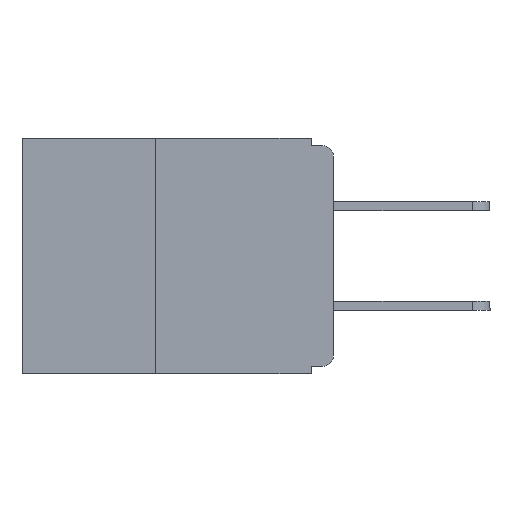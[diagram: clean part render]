
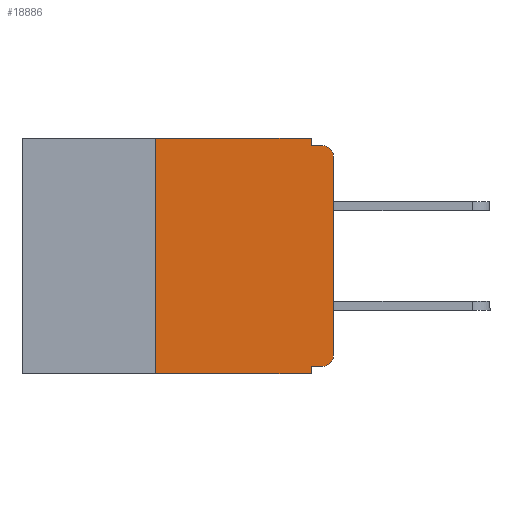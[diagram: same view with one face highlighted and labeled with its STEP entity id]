
A CAD part, left-side view. The second image highlights one B-rep face of the part: STEP entity #18886.
In plain terms, the highlighted planar face has unit normal (-1, 0, 0).
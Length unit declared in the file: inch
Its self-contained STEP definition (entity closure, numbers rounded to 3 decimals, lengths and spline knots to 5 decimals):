
#1476 = EDGE_CURVE ( 'NONE', #25379, #18260, #19982, .T. ) ;
#1733 = VECTOR ( 'NONE', #20077, 39.37008 ) ;
#2137 = CARTESIAN_POINT ( 'NONE',  ( 0., 0.015, -0.025 ) ) ;
#2163 = ORIENTED_EDGE ( 'NONE', *, *, #23606, .F. ) ;
#2522 = ORIENTED_EDGE ( 'NONE', *, *, #3370, .T. ) ;
#3039 = ORIENTED_EDGE ( 'NONE', *, *, #7966, .T. ) ;
#3225 = LINE ( 'NONE', #8152, #17034 ) ;
#3334 = ORIENTED_EDGE ( 'NONE', *, *, #30245, .F. ) ;
#3370 = EDGE_CURVE ( 'NONE', #20870, #31710, #18182, .T. ) ;
#4923 = DIRECTION ( 'NONE',  ( 0., 0., -1. ) ) ;
#5329 = DIRECTION ( 'NONE',  ( 0., 1., 0. ) ) ;
#5519 = DIRECTION ( 'NONE',  ( 0., -1., 0. ) ) ;
#5835 = CARTESIAN_POINT ( 'NONE',  ( 0., 0.437, 0. ) ) ;
#5844 = CARTESIAN_POINT ( 'NONE',  ( 0., 0.25, 0. ) ) ;
#5869 = ORIENTED_EDGE ( 'NONE', *, *, #1476, .F. ) ;
#5966 = VECTOR ( 'NONE', #34291, 39.37008 ) ;
#7051 = CARTESIAN_POINT ( 'NONE',  ( 0., 0.25, -0.33 ) ) ;
#7355 = DIRECTION ( 'NONE',  ( 0., 0., -1. ) ) ;
#7714 = DIRECTION ( 'NONE',  ( 0., -1., 0. ) ) ;
#7966 = EDGE_CURVE ( 'NONE', #30031, #15708, #27254, .T. ) ;
#8152 = CARTESIAN_POINT ( 'NONE',  ( 0., 0., -0.32 ) ) ;
#8555 = CARTESIAN_POINT ( 'NONE',  ( 0., 0.437, -0.33 ) ) ;
#8672 = DIRECTION ( 'NONE',  ( 0., -1., 0. ) ) ;
#9837 = DIRECTION ( 'NONE',  ( 0., 0., 1. ) ) ;
#9908 = CARTESIAN_POINT ( 'NONE',  ( 0., 0.015, -0.32 ) ) ;
#10646 = CARTESIAN_POINT ( 'NONE',  ( 0., 0.437, 0. ) ) ;
#11162 = AXIS2_PLACEMENT_3D ( 'NONE', #10646, #32062, #21606 ) ;
#12258 = DIRECTION ( 'NONE',  ( -1., 0., 0. ) ) ;
#12404 = VERTEX_POINT ( 'NONE', #18757 ) ;
#12510 = VECTOR ( 'NONE', #7355, 39.37008 ) ;
#12816 = CARTESIAN_POINT ( 'NONE',  ( 0., 0.031, -0.01 ) ) ;
#12825 = AXIS2_PLACEMENT_3D ( 'NONE', #2137, #21359, #4923 ) ;
#12866 = VECTOR ( 'NONE', #8672, 39.37008 ) ;
#14148 = VERTEX_POINT ( 'NONE', #17939 ) ;
#14785 = VERTEX_POINT ( 'NONE', #12816 ) ;
#15582 = EDGE_CURVE ( 'NONE', #22468, #20870, #27250, .T. ) ;
#15708 = VERTEX_POINT ( 'NONE', #31457 ) ;
#16165 = PLANE ( 'NONE',  #11162 ) ;
#16212 = CARTESIAN_POINT ( 'NONE',  ( 0., 0.031, 0. ) ) ;
#16541 = EDGE_CURVE ( 'NONE', #22468, #12404, #3225, .T. ) ;
#16612 = CARTESIAN_POINT ( 'NONE',  ( 0., 0., -0.025 ) ) ;
#17034 = VECTOR ( 'NONE', #5329, 39.37008 ) ;
#17939 = CARTESIAN_POINT ( 'NONE',  ( 0., 0.015, -0.01 ) ) ;
#18098 = VECTOR ( 'NONE', #7714, 39.37008 ) ;
#18182 = LINE ( 'NONE', #20532, #1733 ) ;
#18260 = VERTEX_POINT ( 'NONE', #16212 ) ;
#18316 = CARTESIAN_POINT ( 'NONE',  ( 0., 0.031, -0.33 ) ) ;
#18757 = CARTESIAN_POINT ( 'NONE',  ( 0., 0.031, -0.32 ) ) ;
#18886 = ADVANCED_FACE ( 'NONE', ( #21531 ), #16165, .F. ) ;
#18942 = LINE ( 'NONE', #24001, #18098 ) ;
#19369 = EDGE_CURVE ( 'NONE', #18260, #14785, #19815, .T. ) ;
#19815 = LINE ( 'NONE', #26348, #12510 ) ;
#19982 = LINE ( 'NONE', #5835, #27089 ) ;
#20077 = DIRECTION ( 'NONE',  ( 0., 0., 1. ) ) ;
#20402 = VECTOR ( 'NONE', #9837, 39.37008 ) ;
#20460 = ORIENTED_EDGE ( 'NONE', *, *, #31551, .T. ) ;
#20532 = CARTESIAN_POINT ( 'NONE',  ( 0., 0., 0. ) ) ;
#20870 = VERTEX_POINT ( 'NONE', #30432 ) ;
#21359 = DIRECTION ( 'NONE',  ( -1., 0., 0. ) ) ;
#21531 = FACE_OUTER_BOUND ( 'NONE', #27690, .T. ) ;
#21606 = DIRECTION ( 'NONE',  ( 0., 0., -1. ) ) ;
#22468 = VERTEX_POINT ( 'NONE', #9908 ) ;
#22572 = ORIENTED_EDGE ( 'NONE', *, *, #27964, .F. ) ;
#23425 = CIRCLE ( 'NONE', #12825, 0.015 ) ;
#23606 = EDGE_CURVE ( 'NONE', #30031, #25379, #27514, .T. ) ;
#24001 = CARTESIAN_POINT ( 'NONE',  ( 0., 0., -0.01 ) ) ;
#24722 = AXIS2_PLACEMENT_3D ( 'NONE', #28473, #12258, #31125 ) ;
#25379 = VERTEX_POINT ( 'NONE', #5844 ) ;
#26348 = CARTESIAN_POINT ( 'NONE',  ( 0., 0.031, 0. ) ) ;
#26594 = ORIENTED_EDGE ( 'NONE', *, *, #15582, .T. ) ;
#27089 = VECTOR ( 'NONE', #5519, 39.37008 ) ;
#27250 = CIRCLE ( 'NONE', #24722, 0.015 ) ;
#27254 = LINE ( 'NONE', #8555, #12866 ) ;
#27514 = LINE ( 'NONE', #7051, #20402 ) ;
#27690 = EDGE_LOOP ( 'NONE', ( #2522, #20460, #3334, #32537, #5869, #2163, #3039, #22572, #33779, #26594 ) ) ;
#27964 = EDGE_CURVE ( 'NONE', #12404, #15708, #28506, .T. ) ;
#28473 = CARTESIAN_POINT ( 'NONE',  ( 0., 0.015, -0.305 ) ) ;
#28506 = LINE ( 'NONE', #18316, #5966 ) ;
#30031 = VERTEX_POINT ( 'NONE', #31006 ) ;
#30245 = EDGE_CURVE ( 'NONE', #14785, #14148, #18942, .T. ) ;
#30432 = CARTESIAN_POINT ( 'NONE',  ( 0., 0., -0.305 ) ) ;
#31006 = CARTESIAN_POINT ( 'NONE',  ( 0., 0.25, -0.33 ) ) ;
#31125 = DIRECTION ( 'NONE',  ( 0., 0., -1. ) ) ;
#31457 = CARTESIAN_POINT ( 'NONE',  ( 0., 0.031, -0.33 ) ) ;
#31551 = EDGE_CURVE ( 'NONE', #31710, #14148, #23425, .T. ) ;
#31710 = VERTEX_POINT ( 'NONE', #16612 ) ;
#32062 = DIRECTION ( 'NONE',  ( 1., 0., 0. ) ) ;
#32537 = ORIENTED_EDGE ( 'NONE', *, *, #19369, .F. ) ;
#33779 = ORIENTED_EDGE ( 'NONE', *, *, #16541, .F. ) ;
#34291 = DIRECTION ( 'NONE',  ( 0., 0., -1. ) ) ;
